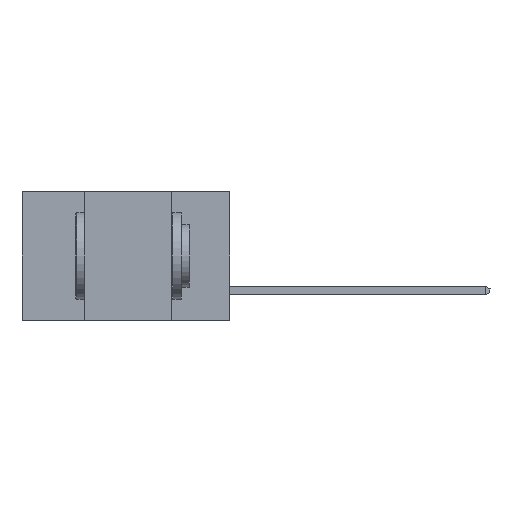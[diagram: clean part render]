
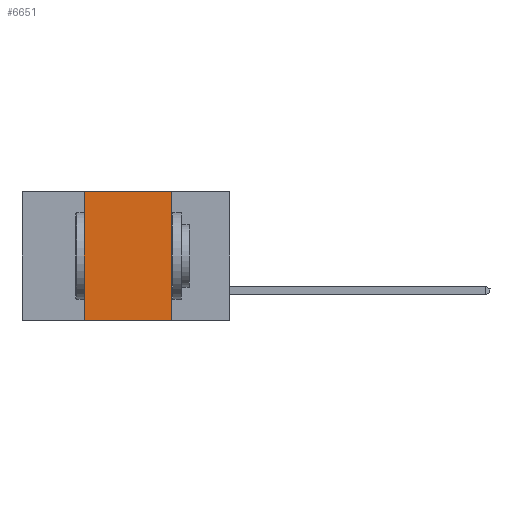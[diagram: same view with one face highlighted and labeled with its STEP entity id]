
A CAD part, left-side view. The second image highlights one B-rep face of the part: STEP entity #6651.
In plain terms, the highlighted planar face has unit normal (-1, 0, 0).
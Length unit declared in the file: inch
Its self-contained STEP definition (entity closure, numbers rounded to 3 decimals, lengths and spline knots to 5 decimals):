
#202 = FACE_OUTER_BOUND ( 'NONE', #13600, .T. ) ;
#306 = DIRECTION ( 'NONE',  ( 0., 0., 1. ) ) ;
#336 = PLANE ( 'NONE',  #4219 ) ;
#605 = EDGE_CURVE ( 'NONE', #4860, #1973, #6023, .T. ) ;
#623 = VECTOR ( 'NONE', #11369, 39.37008 ) ;
#1424 = LINE ( 'NONE', #12226, #12748 ) ;
#1767 = VERTEX_POINT ( 'NONE', #2854 ) ;
#1973 = VERTEX_POINT ( 'NONE', #8725 ) ;
#2854 = CARTESIAN_POINT ( 'NONE',  ( 0., 0.42, -0.37 ) ) ;
#3139 = ORIENTED_EDGE ( 'NONE', *, *, #10765, .T. ) ;
#3601 = VECTOR ( 'NONE', #7299, 39.37008 ) ;
#3758 = VERTEX_POINT ( 'NONE', #10474 ) ;
#4146 = CARTESIAN_POINT ( 'NONE',  ( 0., 0.6, -0.37 ) ) ;
#4219 = AXIS2_PLACEMENT_3D ( 'NONE', #11057, #8871, #7807 ) ;
#4860 = VERTEX_POINT ( 'NONE', #9894 ) ;
#4940 = ORIENTED_EDGE ( 'NONE', *, *, #605, .F. ) ;
#6023 = LINE ( 'NONE', #7795, #623 ) ;
#6651 = ADVANCED_FACE ( 'NONE', ( #202 ), #336, .F. ) ;
#7299 = DIRECTION ( 'NONE',  ( 0., -1., 0. ) ) ;
#7795 = CARTESIAN_POINT ( 'NONE',  ( 0., 0.6, 0. ) ) ;
#7807 = DIRECTION ( 'NONE',  ( 0., 0., -1. ) ) ;
#7868 = EDGE_CURVE ( 'NONE', #1973, #3758, #1424, .T. ) ;
#8053 = LINE ( 'NONE', #9050, #12234 ) ;
#8725 = CARTESIAN_POINT ( 'NONE',  ( 0., 0.17, 0. ) ) ;
#8871 = DIRECTION ( 'NONE',  ( 1., 0., 0. ) ) ;
#9050 = CARTESIAN_POINT ( 'NONE',  ( 0., 0.42, -0.37 ) ) ;
#9894 = CARTESIAN_POINT ( 'NONE',  ( 0., 0.42, 0. ) ) ;
#10474 = CARTESIAN_POINT ( 'NONE',  ( 0., 0.17, -0.37 ) ) ;
#10765 = EDGE_CURVE ( 'NONE', #1767, #3758, #11469, .T. ) ;
#11057 = CARTESIAN_POINT ( 'NONE',  ( 0., 0.6, 0. ) ) ;
#11160 = DIRECTION ( 'NONE',  ( 0., 0., -1. ) ) ;
#11369 = DIRECTION ( 'NONE',  ( 0., -1., 0. ) ) ;
#11469 = LINE ( 'NONE', #4146, #3601 ) ;
#12202 = ORIENTED_EDGE ( 'NONE', *, *, #7868, .F. ) ;
#12226 = CARTESIAN_POINT ( 'NONE',  ( 0., 0.17, -0.37 ) ) ;
#12234 = VECTOR ( 'NONE', #306, 39.37008 ) ;
#12353 = ORIENTED_EDGE ( 'NONE', *, *, #13628, .F. ) ;
#12748 = VECTOR ( 'NONE', #11160, 39.37008 ) ;
#13600 = EDGE_LOOP ( 'NONE', ( #12202, #4940, #12353, #3139 ) ) ;
#13628 = EDGE_CURVE ( 'NONE', #1767, #4860, #8053, .T. ) ;
